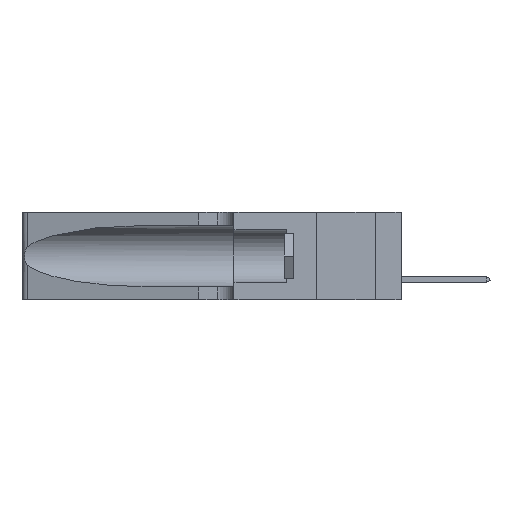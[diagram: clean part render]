
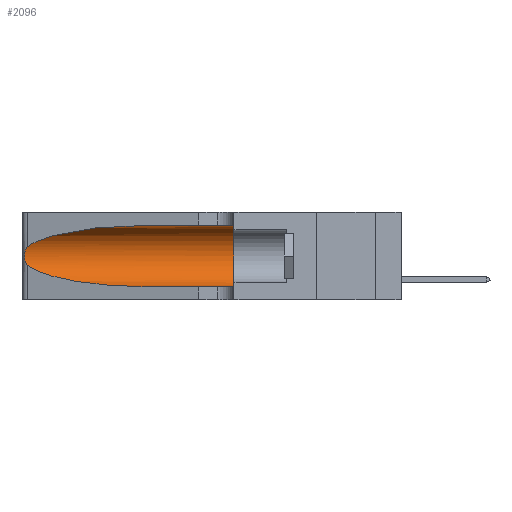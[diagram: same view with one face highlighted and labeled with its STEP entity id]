
A CAD part, left-side view. The second image highlights one B-rep face of the part: STEP entity #2096.
In plain terms, the highlighted cylindrical face has radius 3.308 mm (diameter 6.617 mm), a partial arc.
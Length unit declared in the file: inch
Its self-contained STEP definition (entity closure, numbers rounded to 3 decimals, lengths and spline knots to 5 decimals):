
#320 = DIRECTION ( 'NONE',  ( 0., 0., -1. ) ) ;
#1048 = CARTESIAN_POINT ( 'NONE',  ( 0.26017, 1.23833, 0.17102 ) ) ;
#1167 = CARTESIAN_POINT ( 'NONE',  ( 0.25856, 1.23593, 0.16098 ) ) ;
#1233 = AXIS2_PLACEMENT_3D ( 'NONE', #34187, #29065, #15303 ) ;
#2096 = ADVANCED_FACE ( 'NONE', ( #24248 ), #25119, .F. ) ;
#2889 = DIRECTION ( 'NONE',  ( 0., -1., 0. ) ) ;
#2960 = CARTESIAN_POINT ( 'NONE',  ( 0.1305, 0.35, 0.05475 ) ) ;
#3024 = VECTOR ( 'NONE', #32922, 39.37008 ) ;
#3902 = LINE ( 'NONE', #7971, #3024 ) ;
#3974 = CARTESIAN_POINT ( 'NONE',  ( 0.25487, 1.22718, 0.14631 ) ) ;
#5236 = ORIENTED_EDGE ( 'NONE', *, *, #16166, .T. ) ;
#5357 = CARTESIAN_POINT ( 'NONE',  ( 0.1305, 0.72297, 0.31525 ) ) ;
#6150 =( BOUNDED_CURVE ( )  B_SPLINE_CURVE ( 3, ( #5357, #24539, #30215, #27224 ),
 .UNSPECIFIED., .F., .F. ) 
 B_SPLINE_CURVE_WITH_KNOTS ( ( 4, 4 ),
 ( 1.5708, 2.84003 ),
 .UNSPECIFIED. ) 
 CURVE ( )  GEOMETRIC_REPRESENTATION_ITEM ( )  RATIONAL_B_SPLINE_CURVE ( ( 1., 0.87, 0.87, 1. ) ) 
 REPRESENTATION_ITEM ( '' )  );
#6426 = CARTESIAN_POINT ( 'NONE',  ( 0.25555, 1.22993, 0.14849 ) ) ;
#7971 = CARTESIAN_POINT ( 'NONE',  ( 0.1305, 1.61858, 0.31525 ) ) ;
#8096 = EDGE_CURVE ( 'NONE', #10640, #27314, #28519, .T. ) ;
#8878 = ORIENTED_EDGE ( 'NONE', *, *, #26143, .T. ) ;
#9234 = CARTESIAN_POINT ( 'NONE',  ( 0.1305, 0.72297, 0.05475 ) ) ;
#10640 = VERTEX_POINT ( 'NONE', #13713 ) ;
#10814 = CARTESIAN_POINT ( 'NONE',  ( 0.1305, 0.72297, 0.31525 ) ) ;
#10862 = CARTESIAN_POINT ( 'NONE',  ( 0.1305, 0.72297, 0.05475 ) ) ;
#11940 = CARTESIAN_POINT ( 'NONE',  ( 0.25487, 1.22718, 0.22369 ) ) ;
#12060 = CARTESIAN_POINT ( 'NONE',  ( 0.26075, 1.23896, 0.19203 ) ) ;
#12064 = VERTEX_POINT ( 'NONE', #19716 ) ;
#13703 = EDGE_CURVE ( 'NONE', #21327, #12064, #3902, .T. ) ;
#13713 = CARTESIAN_POINT ( 'NONE',  ( 0.25487, 1.22718, 0.14631 ) ) ;
#14131 = EDGE_LOOP ( 'NONE', ( #29203, #5236, #35177, #8878, #28086, #34963 ) ) ;
#14874 = CARTESIAN_POINT ( 'NONE',  ( 0.25854, 1.2359, 0.20912 ) ) ;
#15015 = CARTESIAN_POINT ( 'NONE',  ( 0.18966, 0.96281, 0.05475 ) ) ;
#15217 = LINE ( 'NONE', #28789, #31596 ) ;
#15303 = DIRECTION ( 'NONE',  ( 0., 0., 1. ) ) ;
#16166 = EDGE_CURVE ( 'NONE', #35029, #10640, #26987, .T. ) ;
#17751 = CARTESIAN_POINT ( 'NONE',  ( 0.26075, 1.23896, 0.178 ) ) ;
#19716 = CARTESIAN_POINT ( 'NONE',  ( 0.1305, 0.35, 0.31525 ) ) ;
#20518 = CARTESIAN_POINT ( 'NONE',  ( 0.25789, 1.23486, 0.15765 ) ) ;
#21327 = VERTEX_POINT ( 'NONE', #10814 ) ;
#21577 = CIRCLE ( 'NONE', #1233, 0.13025 ) ;
#24248 = FACE_OUTER_BOUND ( 'NONE', #14131, .T. ) ;
#24539 = CARTESIAN_POINT ( 'NONE',  ( 0.18966, 0.96281, 0.31525 ) ) ;
#24907 = CARTESIAN_POINT ( 'NONE',  ( 0.1305, 1.61858, 0.185 ) ) ;
#25119 = CYLINDRICAL_SURFACE ( 'NONE', #31222, 0.13025 ) ;
#25731 = CARTESIAN_POINT ( 'NONE',  ( 0.25787, 1.23484, 0.2124 ) ) ;
#25844 = CARTESIAN_POINT ( 'NONE',  ( 0.26018, 1.23835, 0.19895 ) ) ;
#26099 = CARTESIAN_POINT ( 'NONE',  ( 0.25639, 1.23184, 0.21858 ) ) ;
#26143 = EDGE_CURVE ( 'NONE', #27314, #30715, #15217, .T. ) ;
#26987 = B_SPLINE_CURVE_WITH_KNOTS ( 'NONE', 3,
 ( #11940, #34236, #26099, #25731, #14874, #25844, #12060, #17751, #1048, #1167, #20518, #31261, #6426, #3974 ),
 .UNSPECIFIED., .F., .F.,
 ( 4, 2, 2, 2, 2, 2, 4 ),
 ( 0., 0.00027, 0.00053, 0.00107, 0.0016, 0.00187, 0.00214 ),
 .UNSPECIFIED. ) ;
#27224 = CARTESIAN_POINT ( 'NONE',  ( 0.25487, 1.22718, 0.22369 ) ) ;
#27314 = VERTEX_POINT ( 'NONE', #9234 ) ;
#27394 = EDGE_CURVE ( 'NONE', #12064, #30715, #21577, .T. ) ;
#28086 = ORIENTED_EDGE ( 'NONE', *, *, #27394, .F. ) ;
#28319 = DIRECTION ( 'NONE',  ( 0., -1., 0. ) ) ;
#28383 = CARTESIAN_POINT ( 'NONE',  ( 0.25487, 1.22718, 0.22369 ) ) ;
#28519 =( BOUNDED_CURVE ( )  B_SPLINE_CURVE ( 3, ( #33432, #28663, #15015, #10862 ),
 .UNSPECIFIED., .F., .F. ) 
 B_SPLINE_CURVE_WITH_KNOTS ( ( 4, 4 ),
 ( 3.44316, 4.71239 ),
 .UNSPECIFIED. ) 
 CURVE ( )  GEOMETRIC_REPRESENTATION_ITEM ( )  RATIONAL_B_SPLINE_CURVE ( ( 1., 0.87, 0.87, 1. ) ) 
 REPRESENTATION_ITEM ( '' )  );
#28663 = CARTESIAN_POINT ( 'NONE',  ( 0.2373, 1.15595, 0.08982 ) ) ;
#28789 = CARTESIAN_POINT ( 'NONE',  ( 0.1305, 1.61858, 0.05475 ) ) ;
#29065 = DIRECTION ( 'NONE',  ( 0., 1., 0. ) ) ;
#29203 = ORIENTED_EDGE ( 'NONE', *, *, #29820, .T. ) ;
#29820 = EDGE_CURVE ( 'NONE', #21327, #35029, #6150, .T. ) ;
#30215 = CARTESIAN_POINT ( 'NONE',  ( 0.2373, 1.15595, 0.28018 ) ) ;
#30715 = VERTEX_POINT ( 'NONE', #2960 ) ;
#31222 = AXIS2_PLACEMENT_3D ( 'NONE', #24907, #2889, #320 ) ;
#31261 = CARTESIAN_POINT ( 'NONE',  ( 0.25639, 1.23186, 0.15144 ) ) ;
#31596 = VECTOR ( 'NONE', #28319, 39.37008 ) ;
#32922 = DIRECTION ( 'NONE',  ( 0., -1., 0. ) ) ;
#33432 = CARTESIAN_POINT ( 'NONE',  ( 0.25487, 1.22718, 0.14631 ) ) ;
#34187 = CARTESIAN_POINT ( 'NONE',  ( 0.1305, 0.35, 0.185 ) ) ;
#34236 = CARTESIAN_POINT ( 'NONE',  ( 0.25555, 1.22994, 0.2215 ) ) ;
#34963 = ORIENTED_EDGE ( 'NONE', *, *, #13703, .F. ) ;
#35029 = VERTEX_POINT ( 'NONE', #28383 ) ;
#35177 = ORIENTED_EDGE ( 'NONE', *, *, #8096, .T. ) ;
